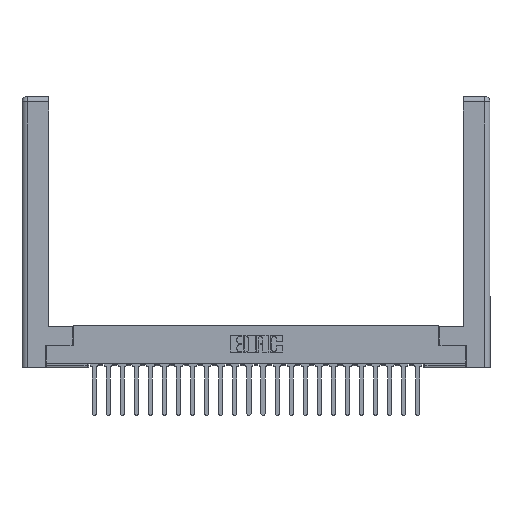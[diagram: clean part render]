
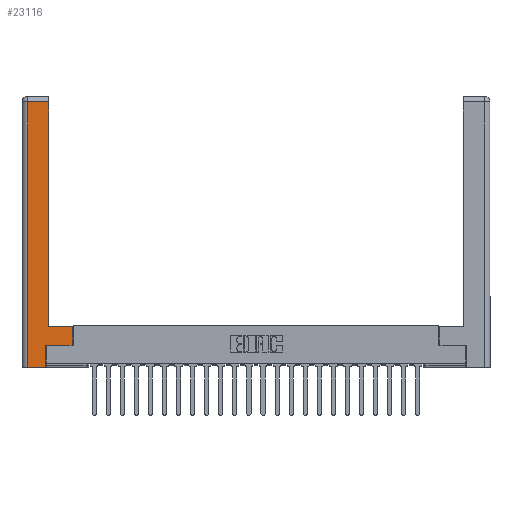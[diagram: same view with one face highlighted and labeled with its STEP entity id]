
A CAD part, top view. The second image highlights one B-rep face of the part: STEP entity #23116.
In plain terms, the highlighted planar face has unit normal (0, 0, 1).
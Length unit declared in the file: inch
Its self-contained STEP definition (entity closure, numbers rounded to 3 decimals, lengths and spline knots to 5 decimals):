
#74 = EDGE_CURVE ( 'NONE', #16211, #3640, #257, .T. ) ;
#257 = LINE ( 'NONE', #7985, #2710 ) ;
#612 = DIRECTION ( 'NONE',  ( 0., 0., -1. ) ) ;
#1400 = DIRECTION ( 'NONE',  ( -1., 0., 0. ) ) ;
#1628 = DIRECTION ( 'NONE',  ( 0., 1., 0. ) ) ;
#2530 = VERTEX_POINT ( 'NONE', #12096 ) ;
#2710 = VECTOR ( 'NONE', #17474, 39.37008 ) ;
#2749 = ORIENTED_EDGE ( 'NONE', *, *, #74, .T. ) ;
#3416 = CARTESIAN_POINT ( 'NONE',  ( 0.265, 0., 0. ) ) ;
#3640 = VERTEX_POINT ( 'NONE', #21638 ) ;
#3755 = ORIENTED_EDGE ( 'NONE', *, *, #16328, .T. ) ;
#4272 = ORIENTED_EDGE ( 'NONE', *, *, #7573, .T. ) ;
#4329 = VERTEX_POINT ( 'NONE', #3416 ) ;
#4453 = DIRECTION ( 'NONE',  ( 1., 0., 0. ) ) ;
#4582 = LINE ( 'NONE', #8456, #8482 ) ;
#4766 = LINE ( 'NONE', #8382, #23035 ) ;
#5717 = VERTEX_POINT ( 'NONE', #19306 ) ;
#5909 = EDGE_CURVE ( 'NONE', #5717, #16211, #24453, .T. ) ;
#6047 = LINE ( 'NONE', #11599, #12351 ) ;
#6122 = LINE ( 'NONE', #9872, #15113 ) ;
#6835 = CARTESIAN_POINT ( 'NONE',  ( 0.565, 0.245, 0. ) ) ;
#7412 = EDGE_CURVE ( 'NONE', #18370, #14734, #6047, .T. ) ;
#7555 = VERTEX_POINT ( 'NONE', #22379 ) ;
#7573 = EDGE_CURVE ( 'NONE', #14734, #2530, #4766, .T. ) ;
#7617 = CARTESIAN_POINT ( 'NONE',  ( 0.0615, 2.94, 0. ) ) ;
#7985 = CARTESIAN_POINT ( 'NONE',  ( 0.565, 0.45, 0. ) ) ;
#8197 = DIRECTION ( 'NONE',  ( 0., 1., 0. ) ) ;
#8382 = CARTESIAN_POINT ( 'NONE',  ( 0.0615, 0., 0. ) ) ;
#8456 = CARTESIAN_POINT ( 'NONE',  ( 0.265, 0., 0. ) ) ;
#8482 = VECTOR ( 'NONE', #4453, 39.37008 ) ;
#8978 = FACE_OUTER_BOUND ( 'NONE', #13158, .T. ) ;
#9872 = CARTESIAN_POINT ( 'NONE',  ( 0.265, 0.245, 0. ) ) ;
#10965 = ORIENTED_EDGE ( 'NONE', *, *, #14093, .T. ) ;
#11206 = CARTESIAN_POINT ( 'NONE',  ( 0.295, 0.45, 0. ) ) ;
#11599 = CARTESIAN_POINT ( 'NONE',  ( 0.0615, 2.94, 0. ) ) ;
#12096 = CARTESIAN_POINT ( 'NONE',  ( 0.0615, 0., 0. ) ) ;
#12351 = VECTOR ( 'NONE', #15685, 39.37008 ) ;
#12581 = ORIENTED_EDGE ( 'NONE', *, *, #7412, .T. ) ;
#12817 = AXIS2_PLACEMENT_3D ( 'NONE', #20273, #612, #24648 ) ;
#13125 = LINE ( 'NONE', #11206, #21255 ) ;
#13158 = EDGE_LOOP ( 'NONE', ( #21635, #12581, #4272, #10965, #17182, #18409, #2749, #3755 ) ) ;
#14028 = CARTESIAN_POINT ( 'NONE',  ( 0.565, 0.245, 0. ) ) ;
#14093 = EDGE_CURVE ( 'NONE', #2530, #4329, #4582, .T. ) ;
#14734 = VERTEX_POINT ( 'NONE', #7617 ) ;
#15024 = LINE ( 'NONE', #25299, #18890 ) ;
#15113 = VECTOR ( 'NONE', #8197, 39.37008 ) ;
#15685 = DIRECTION ( 'NONE',  ( -1., 0., 0. ) ) ;
#16211 = VERTEX_POINT ( 'NONE', #14028 ) ;
#16328 = EDGE_CURVE ( 'NONE', #3640, #7555, #13125, .T. ) ;
#16790 = PLANE ( 'NONE',  #12817 ) ;
#16889 = VECTOR ( 'NONE', #18022, 39.37008 ) ;
#17182 = ORIENTED_EDGE ( 'NONE', *, *, #18245, .T. ) ;
#17474 = DIRECTION ( 'NONE',  ( 0., 1., 0. ) ) ;
#18022 = DIRECTION ( 'NONE',  ( 1., 0., 0. ) ) ;
#18245 = EDGE_CURVE ( 'NONE', #4329, #5717, #6122, .T. ) ;
#18370 = VERTEX_POINT ( 'NONE', #18713 ) ;
#18409 = ORIENTED_EDGE ( 'NONE', *, *, #5909, .T. ) ;
#18713 = CARTESIAN_POINT ( 'NONE',  ( 0.295, 2.94, 0. ) ) ;
#18890 = VECTOR ( 'NONE', #1628, 39.37008 ) ;
#19306 = CARTESIAN_POINT ( 'NONE',  ( 0.265, 0.245, 0. ) ) ;
#20273 = CARTESIAN_POINT ( 'NONE',  ( 0., 0., 0. ) ) ;
#21255 = VECTOR ( 'NONE', #1400, 39.37008 ) ;
#21563 = EDGE_CURVE ( 'NONE', #7555, #18370, #15024, .T. ) ;
#21635 = ORIENTED_EDGE ( 'NONE', *, *, #21563, .T. ) ;
#21638 = CARTESIAN_POINT ( 'NONE',  ( 0.565, 0.45, 0. ) ) ;
#22247 = DIRECTION ( 'NONE',  ( 0., -1., 0. ) ) ;
#22379 = CARTESIAN_POINT ( 'NONE',  ( 0.295, 0.45, 0. ) ) ;
#23035 = VECTOR ( 'NONE', #22247, 39.37008 ) ;
#23116 = ADVANCED_FACE ( 'NONE', ( #8978 ), #16790, .F. ) ;
#24453 = LINE ( 'NONE', #6835, #16889 ) ;
#24648 = DIRECTION ( 'NONE',  ( -1., 0., 0. ) ) ;
#25299 = CARTESIAN_POINT ( 'NONE',  ( 0.295, 3., 0. ) ) ;
